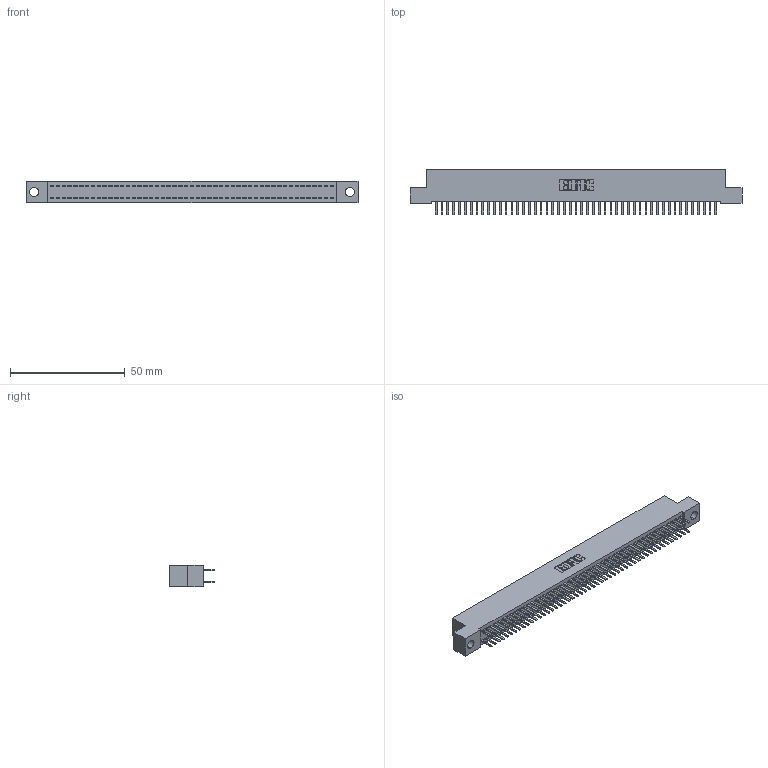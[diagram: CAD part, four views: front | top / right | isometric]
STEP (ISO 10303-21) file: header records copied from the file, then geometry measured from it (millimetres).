
FILE_DESCRIPTION (( 'STEP AP203' ), '1' );
FILE_NAME ('342-098-520-204.STEP', '2019-10-04T16:30:55', ( '' ), ( '' ), 'SwSTEP 2.0', 'SolidWorks 2016', '' );
FILE_SCHEMA (( 'CONFIG_CONTROL_DESIGN' ));
Length unit declared in the file: inch
Products named in the file (3): 342 Part_.156 TH; 345-292-001_345-293-120; 342-098-520-204
Assembly tree (99 placements, depth 2):
  342-098-520-204
    342 Part_.156 TH
    345-292-001_345-293-120  x98
Bounding box: 144.78 x 20.02 x 9.4 mm (x, y, z)
Volume: 12911.5 mm3; surface area: 20911.7 mm2
Topology: 99 solids, 99 shells, 5598 faces, 16273 edges, 10586 vertices
Faces by surface type: plane 3790, cylinder 1808
Entity records: 30603 total; most frequent: CARTESIAN_POINT 5074, ORIENTED_EDGE 4998, DIRECTION 4311, EDGE_CURVE 2499, VECTOR 2367, LINE 2367, VERTEX_POINT 1662, AXIS2_PLACEMENT_3D 972
